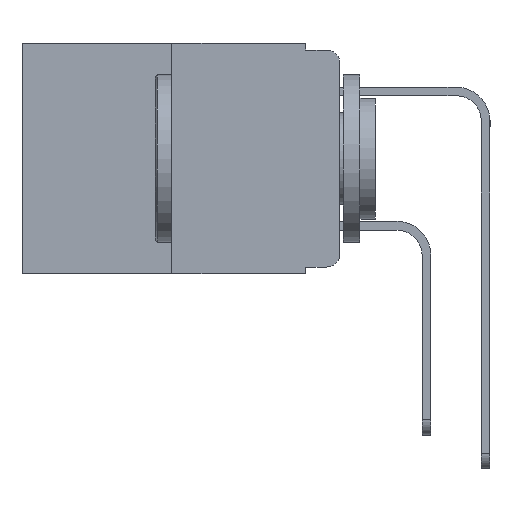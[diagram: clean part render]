
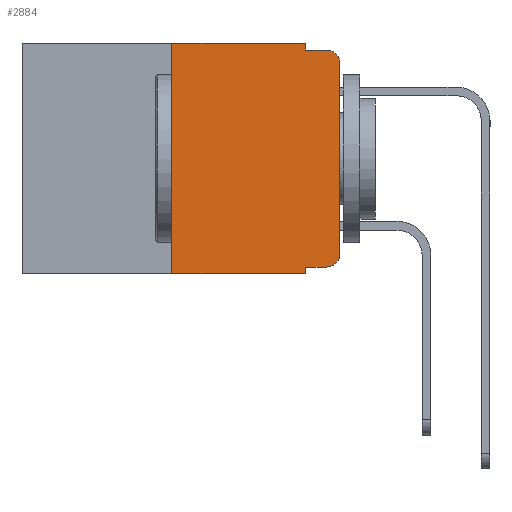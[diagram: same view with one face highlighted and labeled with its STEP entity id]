
A CAD part, left-side view. The second image highlights one B-rep face of the part: STEP entity #2884.
In plain terms, the highlighted planar face has unit normal (-1, 0, 0).
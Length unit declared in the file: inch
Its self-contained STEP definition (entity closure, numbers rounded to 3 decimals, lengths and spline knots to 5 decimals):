
#230 = ORIENTED_EDGE ( 'NONE', *, *, #13864, .T. ) ;
#649 = VERTEX_POINT ( 'NONE', #17710 ) ;
#696 = VERTEX_POINT ( 'NONE', #9943 ) ;
#875 = CARTESIAN_POINT ( 'NONE',  ( 0., 0.051, 0. ) ) ;
#913 = VERTEX_POINT ( 'NONE', #7396 ) ;
#1021 = EDGE_CURVE ( 'NONE', #9942, #913, #13812, .T. ) ;
#1082 = VERTEX_POINT ( 'NONE', #14522 ) ;
#1718 = ORIENTED_EDGE ( 'NONE', *, *, #15527, .F. ) ;
#1827 = LINE ( 'NONE', #6517, #12011 ) ;
#1833 = ORIENTED_EDGE ( 'NONE', *, *, #14908, .T. ) ;
#2349 = LINE ( 'NONE', #2614, #9689 ) ;
#2573 = VERTEX_POINT ( 'NONE', #3937 ) ;
#2582 = DIRECTION ( 'NONE',  ( 0., 0., -1. ) ) ;
#2614 = CARTESIAN_POINT ( 'NONE',  ( 0., 0.051, 0. ) ) ;
#2859 = CARTESIAN_POINT ( 'NONE',  ( 0., 0.051, -0.333 ) ) ;
#2884 = ADVANCED_FACE ( 'NONE', ( #15613 ), #5199, .F. ) ;
#3231 = EDGE_CURVE ( 'NONE', #11270, #913, #13074, .T. ) ;
#3297 = CARTESIAN_POINT ( 'NONE',  ( 0., 0.02, -0.03 ) ) ;
#3320 = DIRECTION ( 'NONE',  ( -1., 0., 0. ) ) ;
#3357 = DIRECTION ( 'NONE',  ( 0., 0., -1. ) ) ;
#3937 = CARTESIAN_POINT ( 'NONE',  ( 0., 0.25, 0. ) ) ;
#3987 = ORIENTED_EDGE ( 'NONE', *, *, #3231, .T. ) ;
#4052 = ORIENTED_EDGE ( 'NONE', *, *, #15946, .F. ) ;
#4392 = DIRECTION ( 'NONE',  ( 0., -1., 0. ) ) ;
#4395 = ORIENTED_EDGE ( 'NONE', *, *, #6206, .T. ) ;
#4617 = CARTESIAN_POINT ( 'NONE',  ( 0., 0.473, 0. ) ) ;
#4748 = ORIENTED_EDGE ( 'NONE', *, *, #1021, .F. ) ;
#5053 = ORIENTED_EDGE ( 'NONE', *, *, #16360, .F. ) ;
#5199 = PLANE ( 'NONE',  #10939 ) ;
#5844 = VECTOR ( 'NONE', #4392, 39.37008 ) ;
#6025 = VECTOR ( 'NONE', #15650, 39.37008 ) ;
#6030 = ORIENTED_EDGE ( 'NONE', *, *, #14692, .T. ) ;
#6206 = EDGE_CURVE ( 'NONE', #1082, #11270, #1827, .T. ) ;
#6481 = LINE ( 'NONE', #14415, #6025 ) ;
#6517 = CARTESIAN_POINT ( 'NONE',  ( 0., 0., 0. ) ) ;
#6960 = LINE ( 'NONE', #15596, #10276 ) ;
#7360 = CARTESIAN_POINT ( 'NONE',  ( 0., 0., -0.03 ) ) ;
#7396 = CARTESIAN_POINT ( 'NONE',  ( 0., 0.02, -0.01 ) ) ;
#8397 = ORIENTED_EDGE ( 'NONE', *, *, #18029, .F. ) ;
#8404 = DIRECTION ( 'NONE',  ( -1., 0., 0. ) ) ;
#8966 = LINE ( 'NONE', #875, #15494 ) ;
#9261 = EDGE_LOOP ( 'NONE', ( #4395, #3987, #4748, #8397, #4052, #5053, #1833, #1718, #6030, #230 ) ) ;
#9401 = VERTEX_POINT ( 'NONE', #9426 ) ;
#9426 = CARTESIAN_POINT ( 'NONE',  ( 0., 0.051, -0.343 ) ) ;
#9689 = VECTOR ( 'NONE', #13850, 39.37008 ) ;
#9942 = VERTEX_POINT ( 'NONE', #13695 ) ;
#9943 = CARTESIAN_POINT ( 'NONE',  ( 0., 0.051, -0.333 ) ) ;
#10068 = LINE ( 'NONE', #2859, #5844 ) ;
#10276 = VECTOR ( 'NONE', #10486, 39.37008 ) ;
#10327 = DIRECTION ( 'NONE',  ( 0., -1., 0. ) ) ;
#10486 = DIRECTION ( 'NONE',  ( 0., -1., 0. ) ) ;
#10538 = VERTEX_POINT ( 'NONE', #16193 ) ;
#10742 = DIRECTION ( 'NONE',  ( 0., 0., 1. ) ) ;
#10832 = AXIS2_PLACEMENT_3D ( 'NONE', #16213, #8404, #17478 ) ;
#10868 = CARTESIAN_POINT ( 'NONE',  ( 0., 0.051, -0.01 ) ) ;
#10939 = AXIS2_PLACEMENT_3D ( 'NONE', #4617, #18085, #17822 ) ;
#11270 = VERTEX_POINT ( 'NONE', #7360 ) ;
#11704 = VERTEX_POINT ( 'NONE', #14757 ) ;
#12011 = VECTOR ( 'NONE', #10742, 39.37008 ) ;
#12063 = AXIS2_PLACEMENT_3D ( 'NONE', #3297, #3320, #3357 ) ;
#12457 = CARTESIAN_POINT ( 'NONE',  ( 0., 0.25, 0. ) ) ;
#12757 = CIRCLE ( 'NONE', #10832, 0.02 ) ;
#13074 = CIRCLE ( 'NONE', #12063, 0.02 ) ;
#13695 = CARTESIAN_POINT ( 'NONE',  ( 0., 0.051, -0.01 ) ) ;
#13812 = LINE ( 'NONE', #10868, #16733 ) ;
#13850 = DIRECTION ( 'NONE',  ( 0., 0., -1. ) ) ;
#13864 = EDGE_CURVE ( 'NONE', #10538, #1082, #12757, .T. ) ;
#14415 = CARTESIAN_POINT ( 'NONE',  ( 0., 0.473, 0. ) ) ;
#14495 = VECTOR ( 'NONE', #16240, 39.37008 ) ;
#14522 = CARTESIAN_POINT ( 'NONE',  ( 0., 0., -0.313 ) ) ;
#14692 = EDGE_CURVE ( 'NONE', #696, #10538, #10068, .T. ) ;
#14757 = CARTESIAN_POINT ( 'NONE',  ( 0., 0.051, 0. ) ) ;
#14880 = LINE ( 'NONE', #12457, #14495 ) ;
#14908 = EDGE_CURVE ( 'NONE', #649, #9401, #6960, .T. ) ;
#15494 = VECTOR ( 'NONE', #2582, 39.37008 ) ;
#15527 = EDGE_CURVE ( 'NONE', #696, #9401, #8966, .T. ) ;
#15596 = CARTESIAN_POINT ( 'NONE',  ( 0., 0.473, -0.343 ) ) ;
#15613 = FACE_OUTER_BOUND ( 'NONE', #9261, .T. ) ;
#15650 = DIRECTION ( 'NONE',  ( 0., -1., 0. ) ) ;
#15946 = EDGE_CURVE ( 'NONE', #2573, #11704, #6481, .T. ) ;
#16193 = CARTESIAN_POINT ( 'NONE',  ( 0., 0.02, -0.333 ) ) ;
#16213 = CARTESIAN_POINT ( 'NONE',  ( 0., 0.02, -0.313 ) ) ;
#16240 = DIRECTION ( 'NONE',  ( 0., 0., 1. ) ) ;
#16360 = EDGE_CURVE ( 'NONE', #649, #2573, #14880, .T. ) ;
#16733 = VECTOR ( 'NONE', #10327, 39.37008 ) ;
#17478 = DIRECTION ( 'NONE',  ( 0., 0., -1. ) ) ;
#17710 = CARTESIAN_POINT ( 'NONE',  ( 0., 0.25, -0.343 ) ) ;
#17822 = DIRECTION ( 'NONE',  ( 0., 0., -1. ) ) ;
#18029 = EDGE_CURVE ( 'NONE', #11704, #9942, #2349, .T. ) ;
#18085 = DIRECTION ( 'NONE',  ( 1., 0., 0. ) ) ;
